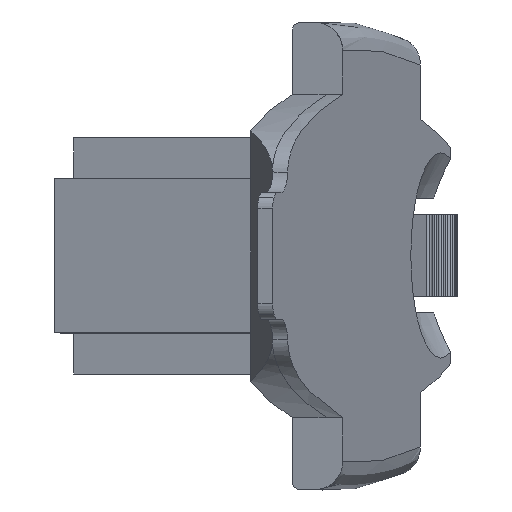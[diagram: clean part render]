
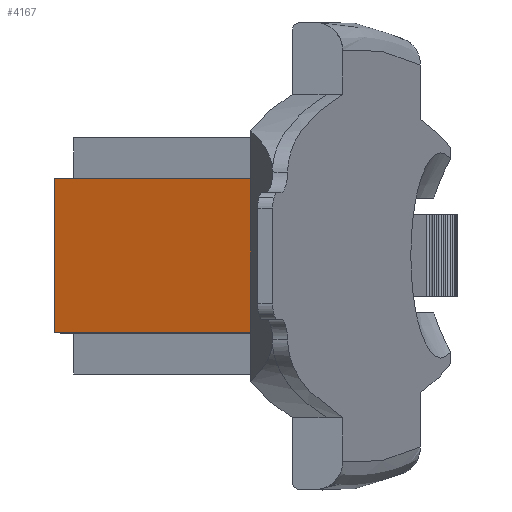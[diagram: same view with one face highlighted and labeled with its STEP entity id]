
A CAD part, left-side view. The second image highlights one B-rep face of the part: STEP entity #4167.
In plain terms, the highlighted planar face has unit normal (-0.945, 0.328, 0).
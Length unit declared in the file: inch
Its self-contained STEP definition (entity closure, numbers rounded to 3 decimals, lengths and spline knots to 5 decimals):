
#27 = LINE ( 'NONE', #5306, #594 ) ;
#28 = CARTESIAN_POINT ( 'NONE',  ( -0.91681, 1.13468, -0.78761 ) ) ;
#35 = EDGE_CURVE ( 'NONE', #162, #5543, #4743, .T. ) ;
#70 = VECTOR ( 'NONE', #5129, 39.37008 ) ;
#162 = VERTEX_POINT ( 'NONE', #3327 ) ;
#193 = LINE ( 'NONE', #2879, #875 ) ;
#233 = VERTEX_POINT ( 'NONE', #595 ) ;
#331 = EDGE_CURVE ( 'NONE', #2534, #5048, #3470, .T. ) ;
#366 = ORIENTED_EDGE ( 'NONE', *, *, #2995, .F. ) ;
#400 = VECTOR ( 'NONE', #3407, 39.37008 ) ;
#429 = CARTESIAN_POINT ( 'NONE',  ( -0.80203, 1.46556, -0.74437 ) ) ;
#555 = CARTESIAN_POINT ( 'NONE',  ( -0.9486, 1.04302, -0.68957 ) ) ;
#557 = DIRECTION ( 'NONE',  ( 0., 0., -1. ) ) ;
#594 = VECTOR ( 'NONE', #3562, 39.37008 ) ;
#595 = CARTESIAN_POINT ( 'NONE',  ( -0.671, 1.84329, -0.68957 ) ) ;
#739 = VECTOR ( 'NONE', #4863, 39.37008 ) ;
#766 = CARTESIAN_POINT ( 'NONE',  ( -0.9486, 1.04302, -0.98497 ) ) ;
#875 = VECTOR ( 'NONE', #3337, 39.37008 ) ;
#893 = ORIENTED_EDGE ( 'NONE', *, *, #922, .T. ) ;
#922 = EDGE_CURVE ( 'NONE', #4901, #162, #969, .T. ) ;
#937 = ORIENTED_EDGE ( 'NONE', *, *, #1679, .T. ) ;
#969 = LINE ( 'NONE', #1471, #739 ) ;
#1047 = PLANE ( 'NONE',  #4170 ) ;
#1109 = LINE ( 'NONE', #766, #400 ) ;
#1421 = EDGE_CURVE ( 'NONE', #233, #3414, #27, .T. ) ;
#1471 = CARTESIAN_POINT ( 'NONE',  ( -0.80205, 1.46551, -1.02783 ) ) ;
#1484 = LINE ( 'NONE', #5514, #1663 ) ;
#1504 = VECTOR ( 'NONE', #2423, 39.37008 ) ;
#1533 = EDGE_CURVE ( 'NONE', #3414, #4538, #193, .T. ) ;
#1581 = VERTEX_POINT ( 'NONE', #4675 ) ;
#1613 = CARTESIAN_POINT ( 'NONE',  ( -0.9486, 1.04302, -0.98497 ) ) ;
#1663 = VECTOR ( 'NONE', #4556, 39.37008 ) ;
#1679 = EDGE_CURVE ( 'NONE', #1581, #4538, #2145, .T. ) ;
#1823 = VECTOR ( 'NONE', #3747, 39.37008 ) ;
#1841 = EDGE_CURVE ( 'NONE', #3356, #233, #5032, .T. ) ;
#1842 = VERTEX_POINT ( 'NONE', #4174 ) ;
#1857 = CARTESIAN_POINT ( 'NONE',  ( -0.671, 1.84329, -0.68957 ) ) ;
#1889 = DIRECTION ( 'NONE',  ( 0.945, -0.328, 0. ) ) ;
#1984 = CARTESIAN_POINT ( 'NONE',  ( -0.80808, 1.44814, -1.08264 ) ) ;
#2107 = CARTESIAN_POINT ( 'NONE',  ( -0.9486, 1.04302, -0.98445 ) ) ;
#2145 = LINE ( 'NONE', #429, #5191 ) ;
#2146 = VECTOR ( 'NONE', #3928, 39.37008 ) ;
#2215 = CARTESIAN_POINT ( 'NONE',  ( -0.671, 1.84329, -1.08279 ) ) ;
#2300 = ORIENTED_EDGE ( 'NONE', *, *, #4165, .T. ) ;
#2326 = ORIENTED_EDGE ( 'NONE', *, *, #2399, .F. ) ;
#2379 = CARTESIAN_POINT ( 'NONE',  ( -0.9486, 1.04302, -1.02775 ) ) ;
#2399 = EDGE_CURVE ( 'NONE', #2534, #3227, #4195, .T. ) ;
#2423 = DIRECTION ( 'NONE',  ( 0., 0., 1. ) ) ;
#2479 = ORIENTED_EDGE ( 'NONE', *, *, #1421, .F. ) ;
#2534 = VERTEX_POINT ( 'NONE', #3440 ) ;
#2566 = CARTESIAN_POINT ( 'NONE',  ( -0.80203, 1.46555, -0.78767 ) ) ;
#2692 = VECTOR ( 'NONE', #2744, 39.37008 ) ;
#2744 = DIRECTION ( 'NONE',  ( -0.002, -0.005, 1. ) ) ;
#2797 = EDGE_CURVE ( 'NONE', #5543, #3227, #1484, .T. ) ;
#2844 = CARTESIAN_POINT ( 'NONE',  ( -0.671, 1.84329, -0.78851 ) ) ;
#2858 = CARTESIAN_POINT ( 'NONE',  ( -0.9165, 1.13557, -0.98446 ) ) ;
#2879 = CARTESIAN_POINT ( 'NONE',  ( -0.9486, 1.04302, -0.98497 ) ) ;
#2995 = EDGE_CURVE ( 'NONE', #1842, #3356, #3724, .T. ) ;
#3071 = VECTOR ( 'NONE', #3922, 39.37008 ) ;
#3227 = VERTEX_POINT ( 'NONE', #2107 ) ;
#3327 = CARTESIAN_POINT ( 'NONE',  ( -0.91643, 1.13576, -1.02777 ) ) ;
#3337 = DIRECTION ( 'NONE',  ( 0., 0., -1. ) ) ;
#3356 = VERTEX_POINT ( 'NONE', #2215 ) ;
#3407 = DIRECTION ( 'NONE',  ( 0., 0., -1. ) ) ;
#3414 = VERTEX_POINT ( 'NONE', #555 ) ;
#3440 = CARTESIAN_POINT ( 'NONE',  ( -0.9486, 1.04302, -0.78759 ) ) ;
#3470 = LINE ( 'NONE', #2566, #2146 ) ;
#3562 = DIRECTION ( 'NONE',  ( -0.328, -0.945, 0. ) ) ;
#3631 = ORIENTED_EDGE ( 'NONE', *, *, #1533, .F. ) ;
#3724 = LINE ( 'NONE', #1984, #70 ) ;
#3747 = DIRECTION ( 'NONE',  ( 0., 0., -1. ) ) ;
#3919 = ORIENTED_EDGE ( 'NONE', *, *, #1841, .F. ) ;
#3922 = DIRECTION ( 'NONE',  ( -0.002, -0.005, 1. ) ) ;
#3928 = DIRECTION ( 'NONE',  ( 0.328, 0.945, 0. ) ) ;
#4011 = ORIENTED_EDGE ( 'NONE', *, *, #4432, .F. ) ;
#4165 = EDGE_CURVE ( 'NONE', #5048, #1581, #5606, .T. ) ;
#4167 = ADVANCED_FACE ( 'NONE', ( #5407 ), #1047, .F. ) ;
#4170 = AXIS2_PLACEMENT_3D ( 'NONE', #1857, #1889, #557 ) ;
#4174 = CARTESIAN_POINT ( 'NONE',  ( -0.9486, 1.04302, -1.08248 ) ) ;
#4195 = LINE ( 'NONE', #1613, #1823 ) ;
#4283 = CARTESIAN_POINT ( 'NONE',  ( -0.91673, 1.13491, -0.83833 ) ) ;
#4432 = EDGE_CURVE ( 'NONE', #4901, #1842, #1109, .T. ) ;
#4483 = ORIENTED_EDGE ( 'NONE', *, *, #35, .T. ) ;
#4538 = VERTEX_POINT ( 'NONE', #5652 ) ;
#4556 = DIRECTION ( 'NONE',  ( -0.328, -0.945, 0. ) ) ;
#4675 = CARTESIAN_POINT ( 'NONE',  ( -0.91688, 1.13448, -0.7443 ) ) ;
#4743 = LINE ( 'NONE', #4283, #3071 ) ;
#4810 = DIRECTION ( 'NONE',  ( -0.328, -0.945, 0. ) ) ;
#4863 = DIRECTION ( 'NONE',  ( 0.328, 0.945, 0. ) ) ;
#4901 = VERTEX_POINT ( 'NONE', #2379 ) ;
#5032 = LINE ( 'NONE', #2844, #1504 ) ;
#5048 = VERTEX_POINT ( 'NONE', #28 ) ;
#5075 = ORIENTED_EDGE ( 'NONE', *, *, #331, .T. ) ;
#5129 = DIRECTION ( 'NONE',  ( 0.328, 0.945, 0. ) ) ;
#5168 = CARTESIAN_POINT ( 'NONE',  ( -0.91688, 1.13446, -0.74039 ) ) ;
#5185 = EDGE_LOOP ( 'NONE', ( #5075, #2300, #937, #3631, #2479, #3919, #366, #4011, #893, #4483, #5644, #2326 ) ) ;
#5191 = VECTOR ( 'NONE', #4810, 39.37008 ) ;
#5306 = CARTESIAN_POINT ( 'NONE',  ( -0.8098, 1.44315, -0.68957 ) ) ;
#5407 = FACE_OUTER_BOUND ( 'NONE', #5185, .T. ) ;
#5514 = CARTESIAN_POINT ( 'NONE',  ( -0.80205, 1.46552, -0.98453 ) ) ;
#5543 = VERTEX_POINT ( 'NONE', #2858 ) ;
#5606 = LINE ( 'NONE', #5168, #2692 ) ;
#5644 = ORIENTED_EDGE ( 'NONE', *, *, #2797, .T. ) ;
#5652 = CARTESIAN_POINT ( 'NONE',  ( -0.9486, 1.04302, -0.74429 ) ) ;
